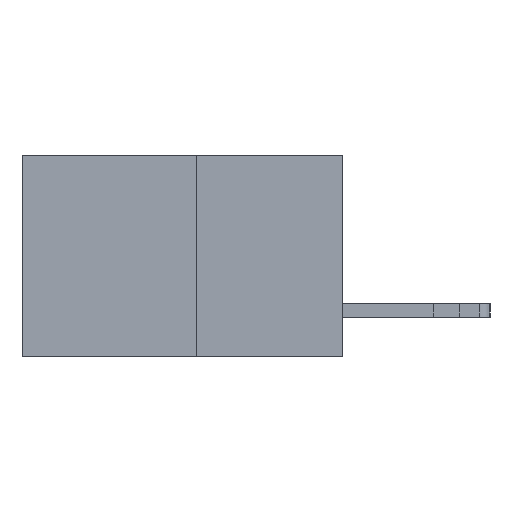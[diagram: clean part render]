
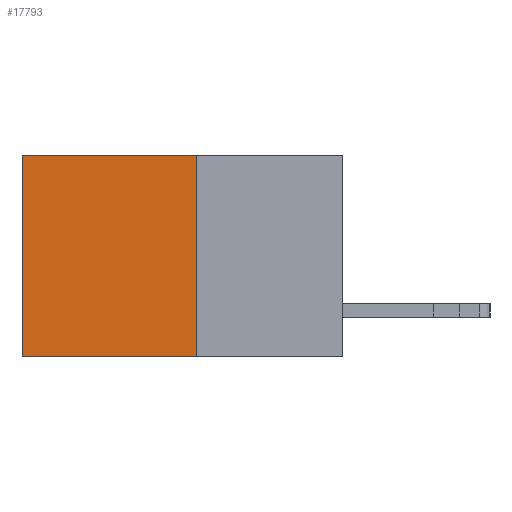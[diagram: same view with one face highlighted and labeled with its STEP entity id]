
A CAD part, left-side view. The second image highlights one B-rep face of the part: STEP entity #17793.
In plain terms, the highlighted planar face has unit normal (-1, 0, 0).
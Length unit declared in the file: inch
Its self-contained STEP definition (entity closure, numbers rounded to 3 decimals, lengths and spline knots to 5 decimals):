
#406 = AXIS2_PLACEMENT_3D ( 'NONE', #13121, #7201, #17542 ) ;
#714 = VERTEX_POINT ( 'NONE', #13840 ) ;
#2209 = EDGE_CURVE ( 'NONE', #18746, #8268, #5024, .T. ) ;
#2984 = LINE ( 'NONE', #12514, #10531 ) ;
#3105 = CARTESIAN_POINT ( 'NONE',  ( 0.277, 0.59, -0.37 ) ) ;
#3988 = EDGE_CURVE ( 'NONE', #714, #18746, #12428, .T. ) ;
#3995 = VECTOR ( 'NONE', #7703, 39.37008 ) ;
#4772 = VERTEX_POINT ( 'NONE', #14316 ) ;
#5024 = LINE ( 'NONE', #10879, #11577 ) ;
#5258 = DIRECTION ( 'NONE',  ( 0., 0., -1. ) ) ;
#6448 = EDGE_LOOP ( 'NONE', ( #13881, #18174, #13053, #7055 ) ) ;
#7055 = ORIENTED_EDGE ( 'NONE', *, *, #3988, .T. ) ;
#7201 = DIRECTION ( 'NONE',  ( 1., 0., 0. ) ) ;
#7703 = DIRECTION ( 'NONE',  ( 0., 1., 0. ) ) ;
#8214 = CARTESIAN_POINT ( 'NONE',  ( 0.277, 0.27, -0.37 ) ) ;
#8268 = VERTEX_POINT ( 'NONE', #3105 ) ;
#8422 = CARTESIAN_POINT ( 'NONE',  ( 0.277, 0.27, 0. ) ) ;
#10531 = VECTOR ( 'NONE', #13973, 39.37008 ) ;
#10534 = EDGE_CURVE ( 'NONE', #4772, #8268, #2984, .T. ) ;
#10879 = CARTESIAN_POINT ( 'NONE',  ( 0.277, 0.59, -0.37 ) ) ;
#11004 = DIRECTION ( 'NONE',  ( 0., 0., -1. ) ) ;
#11406 = FACE_OUTER_BOUND ( 'NONE', #6448, .T. ) ;
#11577 = VECTOR ( 'NONE', #11004, 39.37008 ) ;
#12428 = LINE ( 'NONE', #8422, #3995 ) ;
#12514 = CARTESIAN_POINT ( 'NONE',  ( 0.277, 0.27, -0.37 ) ) ;
#13053 = ORIENTED_EDGE ( 'NONE', *, *, #18881, .F. ) ;
#13121 = CARTESIAN_POINT ( 'NONE',  ( 0.277, 0.27, -0.37 ) ) ;
#13195 = VECTOR ( 'NONE', #5258, 39.37008 ) ;
#13840 = CARTESIAN_POINT ( 'NONE',  ( 0.277, 0.27, 0. ) ) ;
#13881 = ORIENTED_EDGE ( 'NONE', *, *, #2209, .T. ) ;
#13973 = DIRECTION ( 'NONE',  ( 0., 1., 0. ) ) ;
#14316 = CARTESIAN_POINT ( 'NONE',  ( 0.277, 0.27, -0.37 ) ) ;
#15337 = CARTESIAN_POINT ( 'NONE',  ( 0.277, 0.59, 0. ) ) ;
#17542 = DIRECTION ( 'NONE',  ( 0., 0., -1. ) ) ;
#17548 = LINE ( 'NONE', #8214, #13195 ) ;
#17793 = ADVANCED_FACE ( 'NONE', ( #11406 ), #18914, .F. ) ;
#18174 = ORIENTED_EDGE ( 'NONE', *, *, #10534, .F. ) ;
#18746 = VERTEX_POINT ( 'NONE', #15337 ) ;
#18881 = EDGE_CURVE ( 'NONE', #714, #4772, #17548, .T. ) ;
#18914 = PLANE ( 'NONE',  #406 ) ;
